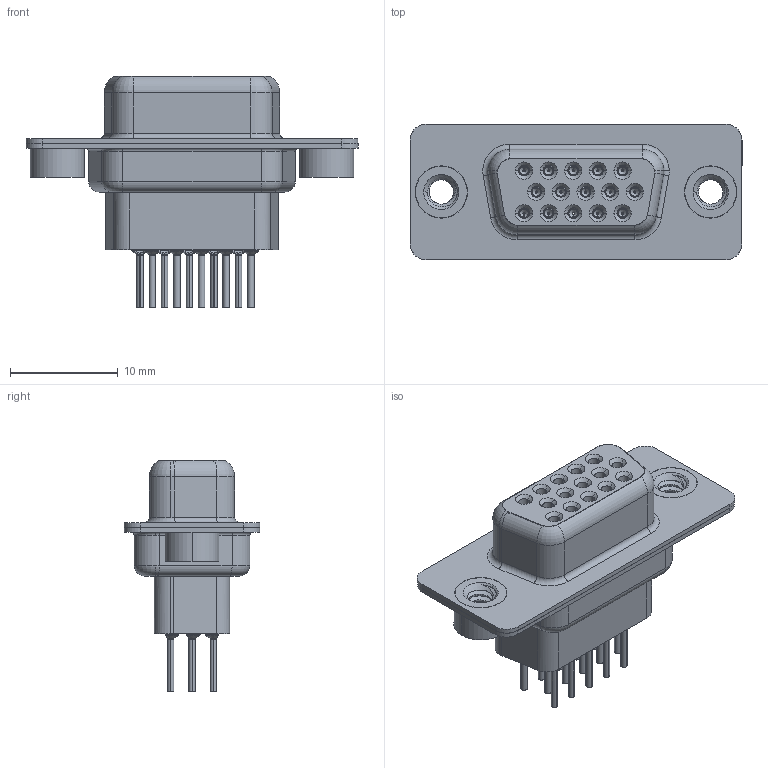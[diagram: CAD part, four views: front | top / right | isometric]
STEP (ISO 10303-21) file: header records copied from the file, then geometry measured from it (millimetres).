
FILE_DESCRIPTION (( 'STEP AP203' ), '1' );
FILE_NAME ('638-015-331-052.STEP', '2019-05-14T18:52:27', ( '' ), ( '' ), 'SwSTEP 2.0', 'SolidWorks 2016', '' );
FILE_SCHEMA (( 'CONFIG_CONTROL_DESIGN' ));
Length unit declared in the file: millimetre
Products named in the file (8): 638-015-331-052; 638 Housing_15 Contacts HP; 638 Shell Front_15 Contacts; 638 Shell Rear_15 Contacts; 638 Contact Row 1_31H; 638 Contact Row 2_31H; 638 Contact Row 3_31H; 638 4-40 Threaded Rivet
Assembly tree (20 placements, depth 2):
  638-015-331-052
    638 Housing_15 Contacts HP
    638 Shell Front_15 Contacts
    638 Shell Rear_15 Contacts
    638 Contact Row 1_31H  x5
    638 Contact Row 2_31H  x5
    638 Contact Row 3_31H  x5
    638 4-40 Threaded Rivet  x2
Bounding box: 30.81 x 12.6 x 21.5 mm (x, y, z)
Volume: 1883.9 mm3; surface area: 6531.2 mm2
Topology: 20 solids, 20 shells, 2124 faces, 5425 edges, 3382 vertices
Faces by surface type: cylinder 632, plane 532, torus 417, bspline 306, cone 237
Entity records: 28273 total; most frequent: CARTESIAN_POINT 9069, DIRECTION 3840, ORIENTED_EDGE 3770, EDGE_CURVE 1885, AXIS2_PLACEMENT_3D 1592, VERTEX_POINT 1182, EDGE_LOOP 869, CIRCLE 861
